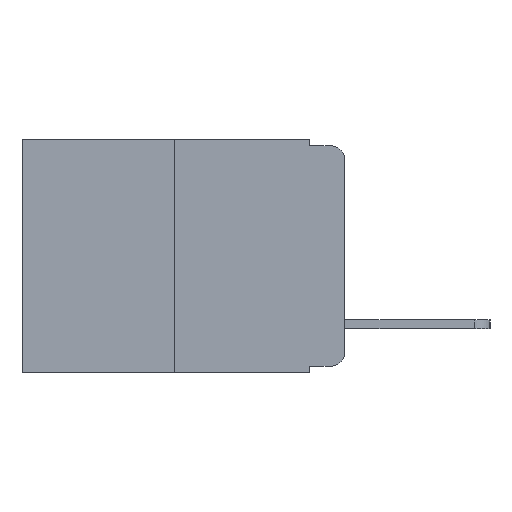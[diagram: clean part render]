
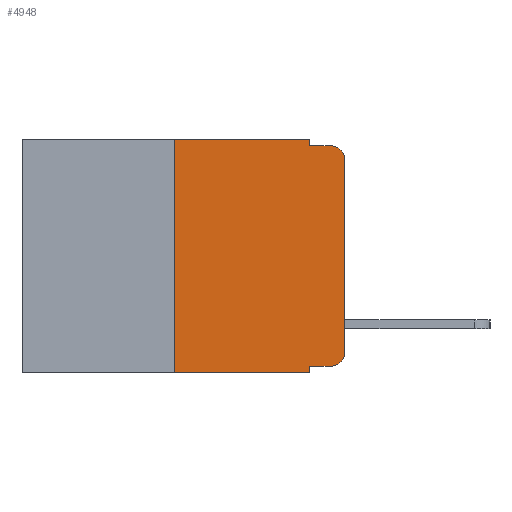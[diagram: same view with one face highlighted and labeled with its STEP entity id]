
A CAD part, left-side view. The second image highlights one B-rep face of the part: STEP entity #4948.
In plain terms, the highlighted planar face has unit normal (-1, 0, 0).
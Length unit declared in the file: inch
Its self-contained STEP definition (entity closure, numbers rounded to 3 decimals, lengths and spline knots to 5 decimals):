
#128 = CARTESIAN_POINT ( 'NONE',  ( 0., 0.051, 0. ) ) ;
#278 = ORIENTED_EDGE ( 'NONE', *, *, #19100, .T. ) ;
#345 = CARTESIAN_POINT ( 'NONE',  ( 0., 0.25, -0.343 ) ) ;
#355 = CARTESIAN_POINT ( 'NONE',  ( 0., 0.473, 0. ) ) ;
#439 = CARTESIAN_POINT ( 'NONE',  ( 0., 0.051, 0. ) ) ;
#829 = ORIENTED_EDGE ( 'NONE', *, *, #2847, .T. ) ;
#1151 = EDGE_CURVE ( 'NONE', #17237, #4485, #18115, .T. ) ;
#1356 = ORIENTED_EDGE ( 'NONE', *, *, #1692, .T. ) ;
#1487 = DIRECTION ( 'NONE',  ( 0., 0., -1. ) ) ;
#1692 = EDGE_CURVE ( 'NONE', #9286, #20383, #6736, .T. ) ;
#1697 = DIRECTION ( 'NONE',  ( 0., -1., 0. ) ) ;
#2147 = DIRECTION ( 'NONE',  ( 0., 0., -1. ) ) ;
#2434 = CARTESIAN_POINT ( 'NONE',  ( 0., 0.25, 0. ) ) ;
#2847 = EDGE_CURVE ( 'NONE', #12868, #9286, #7472, .T. ) ;
#2956 = VERTEX_POINT ( 'NONE', #345 ) ;
#3394 = CARTESIAN_POINT ( 'NONE',  ( 0., 0.25, 0. ) ) ;
#3458 = CARTESIAN_POINT ( 'NONE',  ( 0., 0.051, 0. ) ) ;
#3508 = AXIS2_PLACEMENT_3D ( 'NONE', #3880, #15505, #5594 ) ;
#3574 = AXIS2_PLACEMENT_3D ( 'NONE', #16437, #11595, #1487 ) ;
#3880 = CARTESIAN_POINT ( 'NONE',  ( 0., 0.02, -0.03 ) ) ;
#4028 = VERTEX_POINT ( 'NONE', #8992 ) ;
#4234 = VERTEX_POINT ( 'NONE', #11265 ) ;
#4268 = ORIENTED_EDGE ( 'NONE', *, *, #1151, .F. ) ;
#4485 = VERTEX_POINT ( 'NONE', #3458 ) ;
#4530 = CARTESIAN_POINT ( 'NONE',  ( 0., 0.051, -0.01 ) ) ;
#4609 = VECTOR ( 'NONE', #17693, 39.37008 ) ;
#4948 = ADVANCED_FACE ( 'NONE', ( #17722 ), #9902, .F. ) ;
#5099 = EDGE_CURVE ( 'NONE', #12868, #4234, #11860, .T. ) ;
#5381 = LINE ( 'NONE', #5945, #13718 ) ;
#5385 = CARTESIAN_POINT ( 'NONE',  ( 0., 0.02, -0.313 ) ) ;
#5452 = CIRCLE ( 'NONE', #3508, 0.02 ) ;
#5484 = DIRECTION ( 'NONE',  ( 0., -1., 0. ) ) ;
#5594 = DIRECTION ( 'NONE',  ( 0., 0., -1. ) ) ;
#5945 = CARTESIAN_POINT ( 'NONE',  ( 0., 0.051, -0.01 ) ) ;
#6247 = LINE ( 'NONE', #439, #18395 ) ;
#6248 = EDGE_CURVE ( 'NONE', #2956, #17237, #11044, .T. ) ;
#6521 = CARTESIAN_POINT ( 'NONE',  ( 0., 0., -0.313 ) ) ;
#6736 = CIRCLE ( 'NONE', #17422, 0.02 ) ;
#6891 = VECTOR ( 'NONE', #11951, 39.37008 ) ;
#6948 = VECTOR ( 'NONE', #1697, 39.37008 ) ;
#7099 = DIRECTION ( 'NONE',  ( 0., 0., -1. ) ) ;
#7195 = ORIENTED_EDGE ( 'NONE', *, *, #9627, .F. ) ;
#7385 = EDGE_CURVE ( 'NONE', #4485, #16780, #6247, .T. ) ;
#7472 = LINE ( 'NONE', #10119, #6948 ) ;
#7647 = DIRECTION ( 'NONE',  ( 0., -1., 0. ) ) ;
#7859 = CARTESIAN_POINT ( 'NONE',  ( 0., 0., 0. ) ) ;
#8992 = CARTESIAN_POINT ( 'NONE',  ( 0., 0., -0.03 ) ) ;
#9087 = LINE ( 'NONE', #7859, #4609 ) ;
#9285 = ORIENTED_EDGE ( 'NONE', *, *, #5099, .F. ) ;
#9286 = VERTEX_POINT ( 'NONE', #17125 ) ;
#9627 = EDGE_CURVE ( 'NONE', #16780, #20169, #5381, .T. ) ;
#9902 = PLANE ( 'NONE',  #3574 ) ;
#10119 = CARTESIAN_POINT ( 'NONE',  ( 0., 0.051, -0.333 ) ) ;
#10590 = ORIENTED_EDGE ( 'NONE', *, *, #11864, .T. ) ;
#10753 = EDGE_CURVE ( 'NONE', #4028, #20169, #5452, .T. ) ;
#11044 = LINE ( 'NONE', #3394, #15868 ) ;
#11073 = DIRECTION ( 'NONE',  ( 0., -1., 0. ) ) ;
#11265 = CARTESIAN_POINT ( 'NONE',  ( 0., 0.051, -0.343 ) ) ;
#11595 = DIRECTION ( 'NONE',  ( 1., 0., 0. ) ) ;
#11860 = LINE ( 'NONE', #128, #6891 ) ;
#11864 = EDGE_CURVE ( 'NONE', #20383, #4028, #9087, .T. ) ;
#11951 = DIRECTION ( 'NONE',  ( 0., 0., -1. ) ) ;
#12868 = VERTEX_POINT ( 'NONE', #15770 ) ;
#13166 = ORIENTED_EDGE ( 'NONE', *, *, #6248, .F. ) ;
#13718 = VECTOR ( 'NONE', #7647, 39.37008 ) ;
#13761 = VECTOR ( 'NONE', #5484, 39.37008 ) ;
#15011 = DIRECTION ( 'NONE',  ( 0., 0., 1. ) ) ;
#15505 = DIRECTION ( 'NONE',  ( -1., 0., 0. ) ) ;
#15770 = CARTESIAN_POINT ( 'NONE',  ( 0., 0.051, -0.333 ) ) ;
#15868 = VECTOR ( 'NONE', #15011, 39.37008 ) ;
#15949 = ORIENTED_EDGE ( 'NONE', *, *, #7385, .F. ) ;
#16437 = CARTESIAN_POINT ( 'NONE',  ( 0., 0.473, 0. ) ) ;
#16696 = VECTOR ( 'NONE', #11073, 39.37008 ) ;
#16780 = VERTEX_POINT ( 'NONE', #4530 ) ;
#16967 = DIRECTION ( 'NONE',  ( -1., 0., 0. ) ) ;
#17125 = CARTESIAN_POINT ( 'NONE',  ( 0., 0.02, -0.333 ) ) ;
#17237 = VERTEX_POINT ( 'NONE', #2434 ) ;
#17422 = AXIS2_PLACEMENT_3D ( 'NONE', #5385, #16967, #7099 ) ;
#17693 = DIRECTION ( 'NONE',  ( 0., 0., 1. ) ) ;
#17722 = FACE_OUTER_BOUND ( 'NONE', #21096, .T. ) ;
#18115 = LINE ( 'NONE', #355, #13761 ) ;
#18395 = VECTOR ( 'NONE', #2147, 39.37008 ) ;
#19100 = EDGE_CURVE ( 'NONE', #2956, #4234, #21010, .T. ) ;
#19197 = CARTESIAN_POINT ( 'NONE',  ( 0., 0.473, -0.343 ) ) ;
#19284 = ORIENTED_EDGE ( 'NONE', *, *, #10753, .T. ) ;
#20169 = VERTEX_POINT ( 'NONE', #20767 ) ;
#20383 = VERTEX_POINT ( 'NONE', #6521 ) ;
#20767 = CARTESIAN_POINT ( 'NONE',  ( 0., 0.02, -0.01 ) ) ;
#21010 = LINE ( 'NONE', #19197, #16696 ) ;
#21096 = EDGE_LOOP ( 'NONE', ( #10590, #19284, #7195, #15949, #4268, #13166, #278, #9285, #829, #1356 ) ) ;
